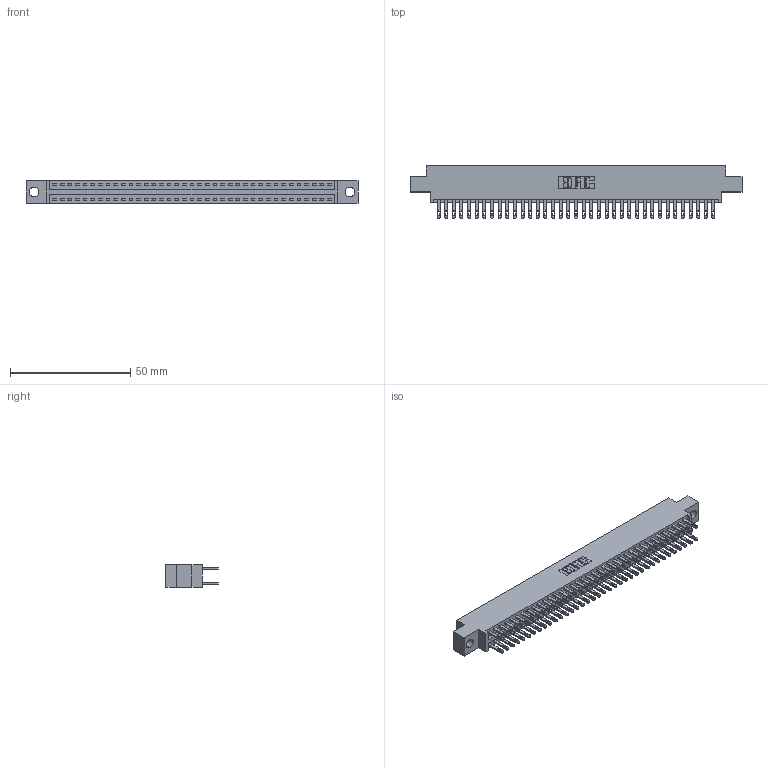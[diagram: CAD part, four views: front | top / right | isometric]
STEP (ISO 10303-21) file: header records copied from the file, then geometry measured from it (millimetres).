
FILE_DESCRIPTION (( 'STEP AP203' ), '1' );
FILE_NAME ('346-074-500-804.STEP', '2018-08-29T01:49:09', ( '' ), ( '' ), 'SwSTEP 2.0', 'SolidWorks 2016', '' );
FILE_SCHEMA (( 'CONFIG_CONTROL_DESIGN' ));
Length unit declared in the file: inch
Products named in the file (3): 345-292-001_345-293-100; 346-074-500-804; 346 Part_0.170 Offset - 0.156 Dia-TH
Assembly tree (75 placements, depth 2):
  346-074-500-804
    346 Part_0.170 Offset - 0.156 Dia-TH
    345-292-001_345-293-100  x74
Bounding box: 138.05 x 21.84 x 9.4 mm (x, y, z)
Volume: 13406.3 mm3; surface area: 19116.8 mm2
Topology: 75 solids, 75 shells, 3678 faces, 11219 edges, 7478 vertices
Faces by surface type: plane 2226, cylinder 1452
Entity records: 24885 total; most frequent: CARTESIAN_POINT 4108, ORIENTED_EDGE 4042, DIRECTION 3673, EDGE_CURVE 2021, VECTOR 1737, LINE 1737, VERTEX_POINT 1346, AXIS2_PLACEMENT_3D 968
